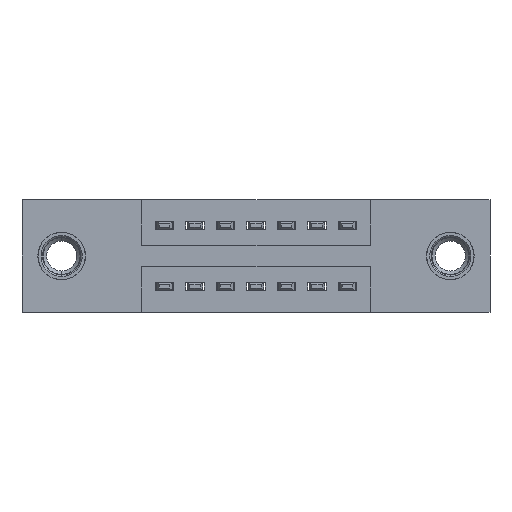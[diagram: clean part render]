
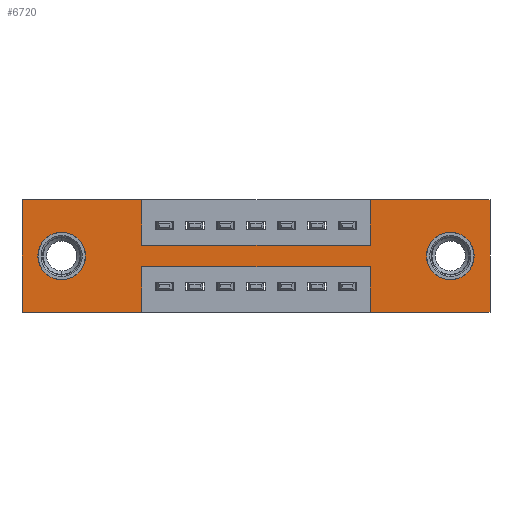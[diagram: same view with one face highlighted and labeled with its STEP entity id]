
A CAD part, front view. The second image highlights one B-rep face of the part: STEP entity #6720.
In plain terms, the highlighted planar face has unit normal (0, -1, 0).
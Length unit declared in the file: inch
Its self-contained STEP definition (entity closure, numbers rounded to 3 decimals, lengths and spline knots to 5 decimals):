
#43 = ORIENTED_EDGE ( 'NONE', *, *, #6089, .F. ) ;
#139 = CARTESIAN_POINT ( 'NONE',  ( 0.13, 0., -0.185 ) ) ;
#171 = EDGE_CURVE ( 'NONE', #3015, #646, #8032, .T. ) ;
#238 = VERTEX_POINT ( 'NONE', #8050 ) ;
#324 = ORIENTED_EDGE ( 'NONE', *, *, #6274, .T. ) ;
#384 = VERTEX_POINT ( 'NONE', #4133 ) ;
#600 = ORIENTED_EDGE ( 'NONE', *, *, #6930, .T. ) ;
#629 = LINE ( 'NONE', #7297, #5321 ) ;
#646 = VERTEX_POINT ( 'NONE', #3827 ) ;
#776 = EDGE_CURVE ( 'NONE', #10816, #6494, #1608, .T. ) ;
#803 = VERTEX_POINT ( 'NONE', #3419 ) ;
#859 = DIRECTION ( 'NONE',  ( 0., 0., -1. ) ) ;
#875 = ORIENTED_EDGE ( 'NONE', *, *, #171, .T. ) ;
#883 = LINE ( 'NONE', #10969, #10172 ) ;
#1037 = DIRECTION ( 'NONE',  ( 0., 0., 1. ) ) ;
#1283 = CARTESIAN_POINT ( 'NONE',  ( 1.405, 0., -0.185 ) ) ;
#1394 = EDGE_CURVE ( 'NONE', #6219, #384, #9540, .T. ) ;
#1486 = CARTESIAN_POINT ( 'NONE',  ( 0.3925, 0., -0.22 ) ) ;
#1499 = AXIS2_PLACEMENT_3D ( 'NONE', #139, #6309, #1037 ) ;
#1577 = ORIENTED_EDGE ( 'NONE', *, *, #9445, .F. ) ;
#1608 = LINE ( 'NONE', #4757, #10835 ) ;
#1748 = CARTESIAN_POINT ( 'NONE',  ( 0.3925, 0., 0. ) ) ;
#1783 = FACE_BOUND ( 'NONE', #8820, .T. ) ;
#1830 = PLANE ( 'NONE',  #5348 ) ;
#1881 = CARTESIAN_POINT ( 'NONE',  ( 0., 0., -0.37 ) ) ;
#1912 = EDGE_CURVE ( 'NONE', #4508, #4243, #2572, .T. ) ;
#1936 = EDGE_CURVE ( 'NONE', #803, #7240, #9254, .T. ) ;
#1966 = EDGE_LOOP ( 'NONE', ( #2973, #875 ) ) ;
#1978 = VECTOR ( 'NONE', #2429, 39.37008 ) ;
#1994 = ORIENTED_EDGE ( 'NONE', *, *, #5737, .F. ) ;
#2032 = DIRECTION ( 'NONE',  ( 0., 0., -1. ) ) ;
#2111 = VECTOR ( 'NONE', #859, 39.37008 ) ;
#2187 = DIRECTION ( 'NONE',  ( 0., 0., -1. ) ) ;
#2291 = VECTOR ( 'NONE', #2481, 39.37008 ) ;
#2429 = DIRECTION ( 'NONE',  ( 0., 0., 1. ) ) ;
#2481 = DIRECTION ( 'NONE',  ( 1., 0., 0. ) ) ;
#2572 = LINE ( 'NONE', #6498, #11168 ) ;
#2697 = CARTESIAN_POINT ( 'NONE',  ( 0., 0., -0.37 ) ) ;
#2795 = CARTESIAN_POINT ( 'NONE',  ( 1.405, 0., -0.107 ) ) ;
#2825 = CARTESIAN_POINT ( 'NONE',  ( 0.3925, 0., -0.37 ) ) ;
#2915 = CARTESIAN_POINT ( 'NONE',  ( 1.1425, 0., -0.22 ) ) ;
#2973 = ORIENTED_EDGE ( 'NONE', *, *, #5445, .T. ) ;
#3015 = VERTEX_POINT ( 'NONE', #5329 ) ;
#3090 = VERTEX_POINT ( 'NONE', #5398 ) ;
#3419 = CARTESIAN_POINT ( 'NONE',  ( 0., 0., -0.37 ) ) ;
#3527 = VECTOR ( 'NONE', #6744, 39.37008 ) ;
#3614 = DIRECTION ( 'NONE',  ( 0., 0., -1. ) ) ;
#3668 = DIRECTION ( 'NONE',  ( -1., 0., 0. ) ) ;
#3798 = ORIENTED_EDGE ( 'NONE', *, *, #4649, .F. ) ;
#3803 = LINE ( 'NONE', #1486, #3527 ) ;
#3827 = CARTESIAN_POINT ( 'NONE',  ( 0.13, 0., -0.107 ) ) ;
#3874 = FACE_BOUND ( 'NONE', #1966, .T. ) ;
#3914 = EDGE_CURVE ( 'NONE', #6494, #238, #883, .T. ) ;
#3978 = AXIS2_PLACEMENT_3D ( 'NONE', #1283, #7406, #2187 ) ;
#4066 = DIRECTION ( 'NONE',  ( 1., 0., 0. ) ) ;
#4133 = CARTESIAN_POINT ( 'NONE',  ( 1.1425, 0., -0.37 ) ) ;
#4243 = VERTEX_POINT ( 'NONE', #2825 ) ;
#4297 = AXIS2_PLACEMENT_3D ( 'NONE', #8015, #7995, #7948 ) ;
#4438 = LINE ( 'NONE', #10128, #4718 ) ;
#4508 = VERTEX_POINT ( 'NONE', #6645 ) ;
#4649 = EDGE_CURVE ( 'NONE', #384, #5526, #11142, .T. ) ;
#4718 = VECTOR ( 'NONE', #4066, 39.37008 ) ;
#4757 = CARTESIAN_POINT ( 'NONE',  ( 0.3925, 0., -0.15 ) ) ;
#4785 = DIRECTION ( 'NONE',  ( 0., 1., 0. ) ) ;
#4818 = DIRECTION ( 'NONE',  ( 1., 0., 0. ) ) ;
#4831 = EDGE_CURVE ( 'NONE', #5385, #10816, #8806, .T. ) ;
#4923 = VECTOR ( 'NONE', #9425, 39.37008 ) ;
#5321 = VECTOR ( 'NONE', #2032, 39.37008 ) ;
#5329 = CARTESIAN_POINT ( 'NONE',  ( 0.13, 0., -0.263 ) ) ;
#5348 = AXIS2_PLACEMENT_3D ( 'NONE', #2697, #6209, #3614 ) ;
#5385 = VERTEX_POINT ( 'NONE', #8775 ) ;
#5388 = CIRCLE ( 'NONE', #1499, 0.078 ) ;
#5398 = CARTESIAN_POINT ( 'NONE',  ( 1.535, 0., 0. ) ) ;
#5445 = EDGE_CURVE ( 'NONE', #646, #3015, #5388, .T. ) ;
#5506 = VECTOR ( 'NONE', #3668, 39.37008 ) ;
#5526 = VERTEX_POINT ( 'NONE', #2915 ) ;
#5737 = EDGE_CURVE ( 'NONE', #238, #3090, #4438, .T. ) ;
#5829 = ORIENTED_EDGE ( 'NONE', *, *, #10012, .F. ) ;
#5844 = DIRECTION ( 'NONE',  ( 0., 0., 1. ) ) ;
#5904 = CARTESIAN_POINT ( 'NONE',  ( 1.1425, 0., -0.15 ) ) ;
#6089 = EDGE_CURVE ( 'NONE', #4243, #803, #9842, .T. ) ;
#6181 = FACE_OUTER_BOUND ( 'NONE', #7693, .T. ) ;
#6209 = DIRECTION ( 'NONE',  ( 0., -1., 0. ) ) ;
#6219 = VERTEX_POINT ( 'NONE', #7267 ) ;
#6274 = EDGE_CURVE ( 'NONE', #7430, #8613, #10749, .T. ) ;
#6309 = DIRECTION ( 'NONE',  ( 0., 1., 0. ) ) ;
#6494 = VERTEX_POINT ( 'NONE', #5904 ) ;
#6498 = CARTESIAN_POINT ( 'NONE',  ( 0.3925, 0., -0.37 ) ) ;
#6537 = CARTESIAN_POINT ( 'NONE',  ( 0., 0., 0. ) ) ;
#6645 = CARTESIAN_POINT ( 'NONE',  ( 0.3925, 0., -0.22 ) ) ;
#6720 = ADVANCED_FACE ( 'NONE', ( #1783, #3874, #6181 ), #1830, .T. ) ;
#6744 = DIRECTION ( 'NONE',  ( -1., 0., 0. ) ) ;
#6794 = ORIENTED_EDGE ( 'NONE', *, *, #1936, .F. ) ;
#6910 = CARTESIAN_POINT ( 'NONE',  ( 0., 0., 0. ) ) ;
#6930 = EDGE_CURVE ( 'NONE', #8613, #7430, #8337, .T. ) ;
#7240 = VERTEX_POINT ( 'NONE', #6910 ) ;
#7267 = CARTESIAN_POINT ( 'NONE',  ( 1.535, 0., -0.37 ) ) ;
#7297 = CARTESIAN_POINT ( 'NONE',  ( 1.535, 0., 0. ) ) ;
#7406 = DIRECTION ( 'NONE',  ( 0., 1., 0. ) ) ;
#7430 = VERTEX_POINT ( 'NONE', #2795 ) ;
#7533 = AXIS2_PLACEMENT_3D ( 'NONE', #9956, #4785, #10784 ) ;
#7626 = CARTESIAN_POINT ( 'NONE',  ( 0.3925, 0., -0.15 ) ) ;
#7655 = CARTESIAN_POINT ( 'NONE',  ( 1.1425, 0., -0.37 ) ) ;
#7693 = EDGE_LOOP ( 'NONE', ( #7868, #5829, #3798, #8409, #8687, #1994, #11155, #9766, #7994, #1577, #6794, #43 ) ) ;
#7868 = ORIENTED_EDGE ( 'NONE', *, *, #1912, .F. ) ;
#7948 = DIRECTION ( 'NONE',  ( 0., 0., 1. ) ) ;
#7994 = ORIENTED_EDGE ( 'NONE', *, *, #4831, .F. ) ;
#7995 = DIRECTION ( 'NONE',  ( 0., 1., 0. ) ) ;
#8015 = CARTESIAN_POINT ( 'NONE',  ( 0.13, 0., -0.185 ) ) ;
#8032 = CIRCLE ( 'NONE', #4297, 0.078 ) ;
#8050 = CARTESIAN_POINT ( 'NONE',  ( 1.1425, 0., 0. ) ) ;
#8337 = CIRCLE ( 'NONE', #3978, 0.078 ) ;
#8409 = ORIENTED_EDGE ( 'NONE', *, *, #1394, .F. ) ;
#8594 = EDGE_CURVE ( 'NONE', #3090, #6219, #629, .T. ) ;
#8613 = VERTEX_POINT ( 'NONE', #10738 ) ;
#8687 = ORIENTED_EDGE ( 'NONE', *, *, #8594, .F. ) ;
#8775 = CARTESIAN_POINT ( 'NONE',  ( 0.3925, 0., 0. ) ) ;
#8806 = LINE ( 'NONE', #1748, #2111 ) ;
#8820 = EDGE_LOOP ( 'NONE', ( #324, #600 ) ) ;
#9115 = DIRECTION ( 'NONE',  ( 0., 0., -1. ) ) ;
#9254 = LINE ( 'NONE', #6537, #10937 ) ;
#9258 = LINE ( 'NONE', #10300, #2291 ) ;
#9425 = DIRECTION ( 'NONE',  ( -1., 0., 0. ) ) ;
#9439 = CARTESIAN_POINT ( 'NONE',  ( 0., 0., -0.37 ) ) ;
#9445 = EDGE_CURVE ( 'NONE', #7240, #5385, #9258, .T. ) ;
#9540 = LINE ( 'NONE', #9439, #4923 ) ;
#9766 = ORIENTED_EDGE ( 'NONE', *, *, #776, .F. ) ;
#9842 = LINE ( 'NONE', #1881, #5506 ) ;
#9956 = CARTESIAN_POINT ( 'NONE',  ( 1.405, 0., -0.185 ) ) ;
#10012 = EDGE_CURVE ( 'NONE', #5526, #4508, #3803, .T. ) ;
#10128 = CARTESIAN_POINT ( 'NONE',  ( 0., 0., 0. ) ) ;
#10172 = VECTOR ( 'NONE', #5844, 39.37008 ) ;
#10300 = CARTESIAN_POINT ( 'NONE',  ( 0., 0., 0. ) ) ;
#10738 = CARTESIAN_POINT ( 'NONE',  ( 1.405, 0., -0.263 ) ) ;
#10749 = CIRCLE ( 'NONE', #7533, 0.078 ) ;
#10784 = DIRECTION ( 'NONE',  ( 0., 0., -1. ) ) ;
#10796 = DIRECTION ( 'NONE',  ( 0., 0., 1. ) ) ;
#10816 = VERTEX_POINT ( 'NONE', #7626 ) ;
#10835 = VECTOR ( 'NONE', #4818, 39.37008 ) ;
#10937 = VECTOR ( 'NONE', #10796, 39.37008 ) ;
#10969 = CARTESIAN_POINT ( 'NONE',  ( 1.1425, 0., 0. ) ) ;
#11142 = LINE ( 'NONE', #7655, #1978 ) ;
#11155 = ORIENTED_EDGE ( 'NONE', *, *, #3914, .F. ) ;
#11168 = VECTOR ( 'NONE', #9115, 39.37008 ) ;
